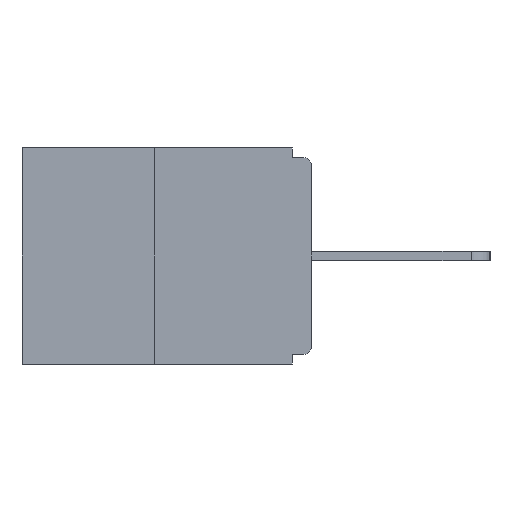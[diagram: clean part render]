
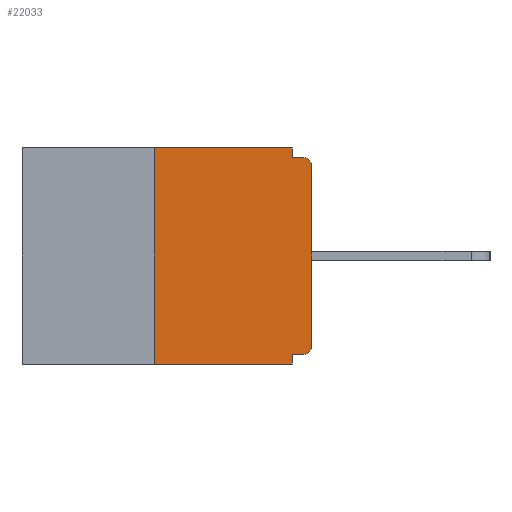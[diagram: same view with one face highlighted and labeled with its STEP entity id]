
A CAD part, left-side view. The second image highlights one B-rep face of the part: STEP entity #22033.
In plain terms, the highlighted planar face has unit normal (-1, 0, 0).
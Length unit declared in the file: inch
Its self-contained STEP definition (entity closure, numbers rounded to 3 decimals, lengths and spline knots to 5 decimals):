
#281 = DIRECTION ( 'NONE',  ( 0., 1., 0. ) ) ;
#693 = CARTESIAN_POINT ( 'NONE',  ( 0., 0.031, -0.015 ) ) ;
#1382 = ORIENTED_EDGE ( 'NONE', *, *, #15413, .T. ) ;
#1687 = DIRECTION ( 'NONE',  ( 0., 0., 1. ) ) ;
#1846 = CARTESIAN_POINT ( 'NONE',  ( 0., 0.031, 0. ) ) ;
#1943 = CIRCLE ( 'NONE', #8683, 0.015 ) ;
#1951 = DIRECTION ( 'NONE',  ( 0., -1., 0. ) ) ;
#1986 = VECTOR ( 'NONE', #13317, 39.37008 ) ;
#3416 = CARTESIAN_POINT ( 'NONE',  ( 0., 0.031, -0.328 ) ) ;
#3875 = CARTESIAN_POINT ( 'NONE',  ( 0., 0.015, -0.328 ) ) ;
#4136 = CARTESIAN_POINT ( 'NONE',  ( 0., 0., -0.313 ) ) ;
#4689 = EDGE_CURVE ( 'NONE', #8364, #21051, #19792, .T. ) ;
#5023 = VERTEX_POINT ( 'NONE', #9314 ) ;
#5132 = EDGE_CURVE ( 'NONE', #17905, #16428, #25699, .T. ) ;
#5234 = VERTEX_POINT ( 'NONE', #3875 ) ;
#5382 = CARTESIAN_POINT ( 'NONE',  ( 0., 0.25, -0.343 ) ) ;
#5635 = CARTESIAN_POINT ( 'NONE',  ( 0., 0., -0.015 ) ) ;
#5833 = DIRECTION ( 'NONE',  ( 0., 0., -1. ) ) ;
#6160 = CARTESIAN_POINT ( 'NONE',  ( 0., 0., -0.03 ) ) ;
#6525 = ORIENTED_EDGE ( 'NONE', *, *, #13830, .F. ) ;
#6762 = PLANE ( 'NONE',  #21140 ) ;
#6975 = ORIENTED_EDGE ( 'NONE', *, *, #5132, .F. ) ;
#7956 = EDGE_CURVE ( 'NONE', #24896, #14523, #8001, .T. ) ;
#8001 = LINE ( 'NONE', #14068, #9859 ) ;
#8317 = AXIS2_PLACEMENT_3D ( 'NONE', #17712, #26015, #17585 ) ;
#8323 = LINE ( 'NONE', #12284, #20003 ) ;
#8364 = VERTEX_POINT ( 'NONE', #4136 ) ;
#8605 = DIRECTION ( 'NONE',  ( 1., 0., 0. ) ) ;
#8683 = AXIS2_PLACEMENT_3D ( 'NONE', #21700, #25788, #5833 ) ;
#9314 = CARTESIAN_POINT ( 'NONE',  ( 0., 0.015, -0.015 ) ) ;
#9749 = LINE ( 'NONE', #5635, #19379 ) ;
#9859 = VECTOR ( 'NONE', #24128, 39.37008 ) ;
#9916 = EDGE_CURVE ( 'NONE', #5234, #8364, #1943, .T. ) ;
#10690 = CARTESIAN_POINT ( 'NONE',  ( 0., 0.25, 0. ) ) ;
#11617 = VERTEX_POINT ( 'NONE', #10690 ) ;
#12284 = CARTESIAN_POINT ( 'NONE',  ( 0., 0., -0.328 ) ) ;
#12732 = EDGE_LOOP ( 'NONE', ( #24577, #19869, #1382, #15238, #6525, #23428, #21335, #17287, #24731, #6975 ) ) ;
#13317 = DIRECTION ( 'NONE',  ( 0., 0., 1. ) ) ;
#13534 = DIRECTION ( 'NONE',  ( 0., 0., -1. ) ) ;
#13830 = EDGE_CURVE ( 'NONE', #5234, #24896, #8323, .T. ) ;
#14068 = CARTESIAN_POINT ( 'NONE',  ( 0., 0.031, -0.343 ) ) ;
#14523 = VERTEX_POINT ( 'NONE', #18296 ) ;
#14895 = CARTESIAN_POINT ( 'NONE',  ( 0., 0.25, 0. ) ) ;
#15238 = ORIENTED_EDGE ( 'NONE', *, *, #7956, .F. ) ;
#15413 = EDGE_CURVE ( 'NONE', #18301, #14523, #16804, .T. ) ;
#16428 = VERTEX_POINT ( 'NONE', #693 ) ;
#16736 = EDGE_CURVE ( 'NONE', #21051, #5023, #17192, .T. ) ;
#16804 = LINE ( 'NONE', #24850, #21780 ) ;
#17001 = EDGE_CURVE ( 'NONE', #18301, #11617, #17020, .T. ) ;
#17020 = LINE ( 'NONE', #14895, #1986 ) ;
#17067 = DIRECTION ( 'NONE',  ( 0., 0., -1. ) ) ;
#17192 = CIRCLE ( 'NONE', #8317, 0.015 ) ;
#17287 = ORIENTED_EDGE ( 'NONE', *, *, #16736, .T. ) ;
#17585 = DIRECTION ( 'NONE',  ( 0., 0., -1. ) ) ;
#17712 = CARTESIAN_POINT ( 'NONE',  ( 0., 0.015, -0.03 ) ) ;
#17905 = VERTEX_POINT ( 'NONE', #1846 ) ;
#18296 = CARTESIAN_POINT ( 'NONE',  ( 0., 0.031, -0.343 ) ) ;
#18301 = VERTEX_POINT ( 'NONE', #5382 ) ;
#18473 = EDGE_CURVE ( 'NONE', #11617, #17905, #20672, .T. ) ;
#19153 = DIRECTION ( 'NONE',  ( 0., -1., 0. ) ) ;
#19379 = VECTOR ( 'NONE', #1951, 39.37008 ) ;
#19792 = LINE ( 'NONE', #23872, #25703 ) ;
#19869 = ORIENTED_EDGE ( 'NONE', *, *, #17001, .F. ) ;
#20003 = VECTOR ( 'NONE', #281, 39.37008 ) ;
#20187 = CARTESIAN_POINT ( 'NONE',  ( 0., 0.46, 0. ) ) ;
#20672 = LINE ( 'NONE', #20187, #23588 ) ;
#20703 = VECTOR ( 'NONE', #13534, 39.37008 ) ;
#20898 = EDGE_CURVE ( 'NONE', #16428, #5023, #9749, .T. ) ;
#21051 = VERTEX_POINT ( 'NONE', #6160 ) ;
#21140 = AXIS2_PLACEMENT_3D ( 'NONE', #24991, #8605, #17067 ) ;
#21335 = ORIENTED_EDGE ( 'NONE', *, *, #4689, .T. ) ;
#21700 = CARTESIAN_POINT ( 'NONE',  ( 0., 0.015, -0.313 ) ) ;
#21780 = VECTOR ( 'NONE', #19153, 39.37008 ) ;
#22033 = ADVANCED_FACE ( 'NONE', ( #22787 ), #6762, .F. ) ;
#22787 = FACE_OUTER_BOUND ( 'NONE', #12732, .T. ) ;
#23428 = ORIENTED_EDGE ( 'NONE', *, *, #9916, .T. ) ;
#23478 = CARTESIAN_POINT ( 'NONE',  ( 0., 0.031, 0. ) ) ;
#23588 = VECTOR ( 'NONE', #24617, 39.37008 ) ;
#23872 = CARTESIAN_POINT ( 'NONE',  ( 0., 0., 0. ) ) ;
#24128 = DIRECTION ( 'NONE',  ( 0., 0., -1. ) ) ;
#24577 = ORIENTED_EDGE ( 'NONE', *, *, #18473, .F. ) ;
#24617 = DIRECTION ( 'NONE',  ( 0., -1., 0. ) ) ;
#24731 = ORIENTED_EDGE ( 'NONE', *, *, #20898, .F. ) ;
#24850 = CARTESIAN_POINT ( 'NONE',  ( 0., 0.46, -0.343 ) ) ;
#24896 = VERTEX_POINT ( 'NONE', #3416 ) ;
#24991 = CARTESIAN_POINT ( 'NONE',  ( 0., 0.46, 0. ) ) ;
#25699 = LINE ( 'NONE', #23478, #20703 ) ;
#25703 = VECTOR ( 'NONE', #1687, 39.37008 ) ;
#25788 = DIRECTION ( 'NONE',  ( -1., 0., 0. ) ) ;
#26015 = DIRECTION ( 'NONE',  ( -1., 0., 0. ) ) ;
